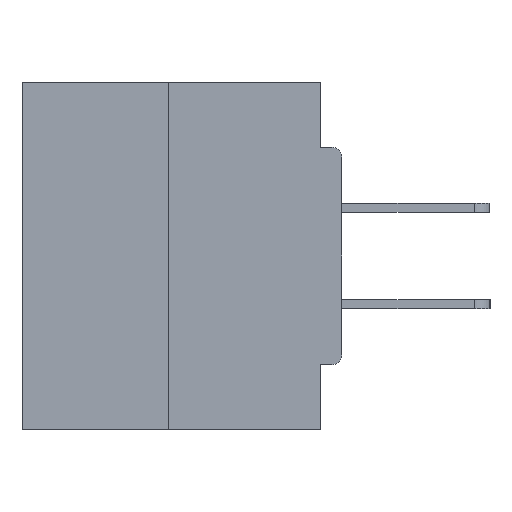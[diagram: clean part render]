
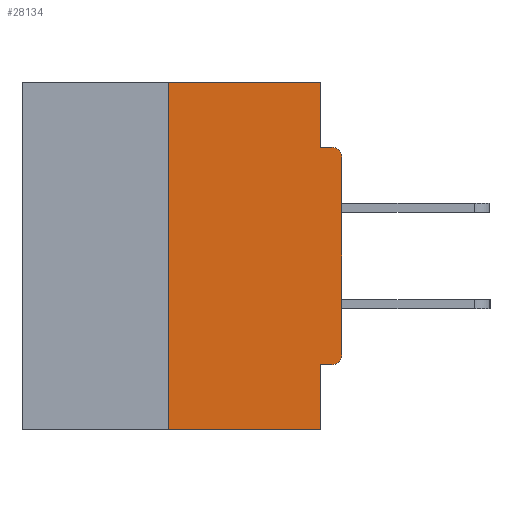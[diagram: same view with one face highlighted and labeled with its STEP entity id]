
A CAD part, left-side view. The second image highlights one B-rep face of the part: STEP entity #28134.
In plain terms, the highlighted planar face has unit normal (-1, 0, 0).
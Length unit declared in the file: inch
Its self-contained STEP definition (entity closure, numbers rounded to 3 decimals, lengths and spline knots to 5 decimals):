
#465 = DIRECTION ( 'NONE',  ( 0., 0., -1. ) ) ;
#648 = DIRECTION ( 'NONE',  ( 1., 0., 0. ) ) ;
#686 = CARTESIAN_POINT ( 'NONE',  ( 0., 0., -0.1085 ) ) ;
#1373 = DIRECTION ( 'NONE',  ( 0., 0., -1. ) ) ;
#1646 = CARTESIAN_POINT ( 'NONE',  ( 0., 0.015, -0.1085 ) ) ;
#2329 = CARTESIAN_POINT ( 'NONE',  ( 0., 0., 0. ) ) ;
#2506 = CARTESIAN_POINT ( 'NONE',  ( 0., 0.031, 0. ) ) ;
#3094 = VERTEX_POINT ( 'NONE', #11751 ) ;
#3336 = VERTEX_POINT ( 'NONE', #9492 ) ;
#3787 = CARTESIAN_POINT ( 'NONE',  ( 0., 0.46, 0. ) ) ;
#4196 = DIRECTION ( 'NONE',  ( 0., 0., -1. ) ) ;
#4332 = ORIENTED_EDGE ( 'NONE', *, *, #41429, .F. ) ;
#4345 = LINE ( 'NONE', #38866, #4889 ) ;
#4889 = VECTOR ( 'NONE', #465, 39.37008 ) ;
#7030 = CARTESIAN_POINT ( 'NONE',  ( 0., 0.46, -0.5 ) ) ;
#7150 = VECTOR ( 'NONE', #25550, 39.37008 ) ;
#8381 = EDGE_CURVE ( 'NONE', #18756, #34574, #4345, .T. ) ;
#8806 = AXIS2_PLACEMENT_3D ( 'NONE', #1646, #11512, #1373 ) ;
#9180 = LINE ( 'NONE', #3787, #7150 ) ;
#9234 = ORIENTED_EDGE ( 'NONE', *, *, #28571, .T. ) ;
#9492 = CARTESIAN_POINT ( 'NONE',  ( 0., 0.015, -0.0935 ) ) ;
#9841 = ORIENTED_EDGE ( 'NONE', *, *, #8381, .F. ) ;
#10701 = DIRECTION ( 'NONE',  ( -1., 0., 0. ) ) ;
#11512 = DIRECTION ( 'NONE',  ( -1., 0., 0. ) ) ;
#11564 = CARTESIAN_POINT ( 'NONE',  ( 0., 0.25, 0. ) ) ;
#11605 = CARTESIAN_POINT ( 'NONE',  ( 0., 0., -0.0935 ) ) ;
#11660 = VERTEX_POINT ( 'NONE', #32462 ) ;
#11751 = CARTESIAN_POINT ( 'NONE',  ( 0., 0.015, -0.4065 ) ) ;
#13275 = DIRECTION ( 'NONE',  ( 0., 1., 0. ) ) ;
#13362 = CARTESIAN_POINT ( 'NONE',  ( 0., 0.46, 0. ) ) ;
#14125 = EDGE_CURVE ( 'NONE', #25688, #18756, #9180, .T. ) ;
#14492 = VECTOR ( 'NONE', #14561, 39.37008 ) ;
#14561 = DIRECTION ( 'NONE',  ( 0., -1., 0. ) ) ;
#15136 = LINE ( 'NONE', #19948, #28663 ) ;
#15374 = CARTESIAN_POINT ( 'NONE',  ( 0., 0.031, -0.5 ) ) ;
#15519 = LINE ( 'NONE', #11605, #14492 ) ;
#17111 = VERTEX_POINT ( 'NONE', #26659 ) ;
#17218 = VECTOR ( 'NONE', #40773, 39.37008 ) ;
#18756 = VERTEX_POINT ( 'NONE', #2506 ) ;
#18996 = VERTEX_POINT ( 'NONE', #35553 ) ;
#19314 = CARTESIAN_POINT ( 'NONE',  ( 0., 0.031, -0.0935 ) ) ;
#19346 = EDGE_CURVE ( 'NONE', #11660, #32125, #23747, .T. ) ;
#19666 = EDGE_CURVE ( 'NONE', #24231, #3336, #27701, .T. ) ;
#19948 = CARTESIAN_POINT ( 'NONE',  ( 0., 0., -0.4065 ) ) ;
#20577 = ORIENTED_EDGE ( 'NONE', *, *, #19346, .F. ) ;
#21419 = LINE ( 'NONE', #2329, #26391 ) ;
#23122 = CIRCLE ( 'NONE', #38554, 0.015 ) ;
#23747 = LINE ( 'NONE', #15374, #17218 ) ;
#24231 = VERTEX_POINT ( 'NONE', #686 ) ;
#24383 = ORIENTED_EDGE ( 'NONE', *, *, #25325, .T. ) ;
#24597 = ORIENTED_EDGE ( 'NONE', *, *, #27539, .F. ) ;
#24692 = FACE_OUTER_BOUND ( 'NONE', #26741, .T. ) ;
#25120 = CARTESIAN_POINT ( 'NONE',  ( 0., 0.031, -0.5 ) ) ;
#25269 = VECTOR ( 'NONE', #36331, 39.37008 ) ;
#25325 = EDGE_CURVE ( 'NONE', #17111, #24231, #21419, .T. ) ;
#25550 = DIRECTION ( 'NONE',  ( 0., -1., 0. ) ) ;
#25688 = VERTEX_POINT ( 'NONE', #11564 ) ;
#26086 = ORIENTED_EDGE ( 'NONE', *, *, #14125, .F. ) ;
#26164 = VECTOR ( 'NONE', #26480, 39.37008 ) ;
#26391 = VECTOR ( 'NONE', #37918, 39.37008 ) ;
#26480 = DIRECTION ( 'NONE',  ( 0., -1., 0. ) ) ;
#26659 = CARTESIAN_POINT ( 'NONE',  ( 0., 0., -0.3915 ) ) ;
#26666 = LINE ( 'NONE', #7030, #26164 ) ;
#26741 = EDGE_LOOP ( 'NONE', ( #26086, #24597, #38342, #20577, #37901, #9234, #24383, #33539, #4332, #9841 ) ) ;
#27539 = EDGE_CURVE ( 'NONE', #18996, #25688, #33708, .T. ) ;
#27701 = CIRCLE ( 'NONE', #8806, 0.015 ) ;
#28088 = EDGE_CURVE ( 'NONE', #18996, #32125, #26666, .T. ) ;
#28134 = ADVANCED_FACE ( 'NONE', ( #24692 ), #35977, .F. ) ;
#28460 = EDGE_CURVE ( 'NONE', #3094, #11660, #15136, .T. ) ;
#28571 = EDGE_CURVE ( 'NONE', #3094, #17111, #23122, .T. ) ;
#28652 = AXIS2_PLACEMENT_3D ( 'NONE', #13362, #648, #4196 ) ;
#28663 = VECTOR ( 'NONE', #13275, 39.37008 ) ;
#29884 = CARTESIAN_POINT ( 'NONE',  ( 0., 0.015, -0.3915 ) ) ;
#32125 = VERTEX_POINT ( 'NONE', #25120 ) ;
#32462 = CARTESIAN_POINT ( 'NONE',  ( 0., 0.031, -0.4065 ) ) ;
#33078 = DIRECTION ( 'NONE',  ( 0., 0., -1. ) ) ;
#33539 = ORIENTED_EDGE ( 'NONE', *, *, #19666, .T. ) ;
#33708 = LINE ( 'NONE', #39412, #25269 ) ;
#34574 = VERTEX_POINT ( 'NONE', #19314 ) ;
#35553 = CARTESIAN_POINT ( 'NONE',  ( 0., 0.25, -0.5 ) ) ;
#35977 = PLANE ( 'NONE',  #28652 ) ;
#36331 = DIRECTION ( 'NONE',  ( 0., 0., 1. ) ) ;
#37901 = ORIENTED_EDGE ( 'NONE', *, *, #28460, .F. ) ;
#37918 = DIRECTION ( 'NONE',  ( 0., 0., 1. ) ) ;
#38342 = ORIENTED_EDGE ( 'NONE', *, *, #28088, .T. ) ;
#38554 = AXIS2_PLACEMENT_3D ( 'NONE', #29884, #10701, #33078 ) ;
#38866 = CARTESIAN_POINT ( 'NONE',  ( 0., 0.031, 0. ) ) ;
#39412 = CARTESIAN_POINT ( 'NONE',  ( 0., 0.25, 0. ) ) ;
#40773 = DIRECTION ( 'NONE',  ( 0., 0., -1. ) ) ;
#41429 = EDGE_CURVE ( 'NONE', #34574, #3336, #15519, .T. ) ;
